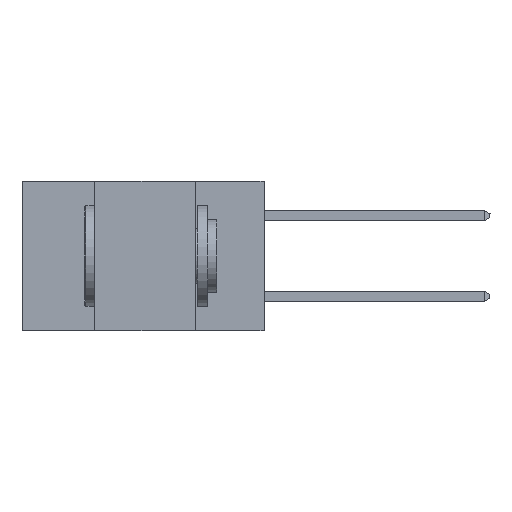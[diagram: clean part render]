
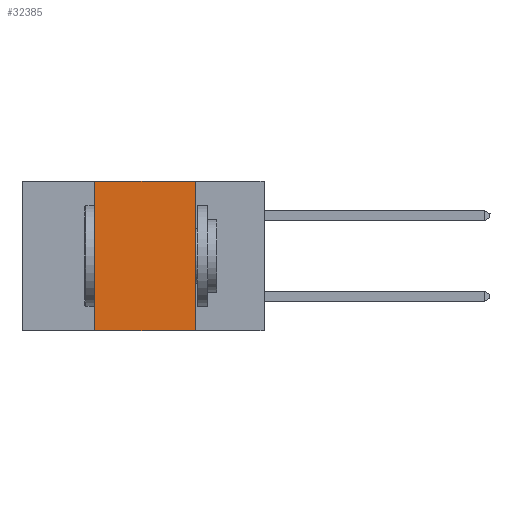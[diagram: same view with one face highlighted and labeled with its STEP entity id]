
A CAD part, left-side view. The second image highlights one B-rep face of the part: STEP entity #32385.
In plain terms, the highlighted planar face has unit normal (-1, 0, 0).
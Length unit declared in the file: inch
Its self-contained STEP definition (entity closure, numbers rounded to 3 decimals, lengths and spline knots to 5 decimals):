
#1073 = AXIS2_PLACEMENT_3D ( 'NONE', #11954, #14558, #14456 ) ;
#1496 = VECTOR ( 'NONE', #25449, 39.37008 ) ;
#1583 = VERTEX_POINT ( 'NONE', #9910 ) ;
#1674 = ORIENTED_EDGE ( 'NONE', *, *, #17111, .F. ) ;
#2244 = DIRECTION ( 'NONE',  ( 0., -1., 0. ) ) ;
#2824 = EDGE_CURVE ( 'NONE', #32663, #30013, #30114, .T. ) ;
#5712 = DIRECTION ( 'NONE',  ( 0., 0., 1. ) ) ;
#8469 = VECTOR ( 'NONE', #2244, 39.37008 ) ;
#8724 = VECTOR ( 'NONE', #5712, 39.37008 ) ;
#9249 = PLANE ( 'NONE',  #1073 ) ;
#9910 = CARTESIAN_POINT ( 'NONE',  ( 0., 0.17, -0.37 ) ) ;
#9993 = ORIENTED_EDGE ( 'NONE', *, *, #13170, .F. ) ;
#10010 = CARTESIAN_POINT ( 'NONE',  ( 0., 0.6, -0.37 ) ) ;
#10573 = CARTESIAN_POINT ( 'NONE',  ( 0., 0.6, 0. ) ) ;
#11084 = ORIENTED_EDGE ( 'NONE', *, *, #2824, .F. ) ;
#11954 = CARTESIAN_POINT ( 'NONE',  ( 0., 0.6, 0. ) ) ;
#13170 = EDGE_CURVE ( 'NONE', #18809, #1583, #32560, .T. ) ;
#14099 = CARTESIAN_POINT ( 'NONE',  ( 0., 0.42, 0. ) ) ;
#14456 = DIRECTION ( 'NONE',  ( 0., 0., -1. ) ) ;
#14558 = DIRECTION ( 'NONE',  ( 1., 0., 0. ) ) ;
#15313 = CARTESIAN_POINT ( 'NONE',  ( 0., 0.42, -0.37 ) ) ;
#15388 = CARTESIAN_POINT ( 'NONE',  ( 0., 0.17, 0. ) ) ;
#17111 = EDGE_CURVE ( 'NONE', #30013, #18809, #28740, .T. ) ;
#17752 = LINE ( 'NONE', #10010, #8469 ) ;
#18809 = VERTEX_POINT ( 'NONE', #15388 ) ;
#20160 = CARTESIAN_POINT ( 'NONE',  ( 0., 0.17, 0. ) ) ;
#21142 = CARTESIAN_POINT ( 'NONE',  ( 0., 0.42, 0. ) ) ;
#23070 = VECTOR ( 'NONE', #31188, 39.37008 ) ;
#25449 = DIRECTION ( 'NONE',  ( 0., 0., -1. ) ) ;
#25602 = FACE_OUTER_BOUND ( 'NONE', #32151, .T. ) ;
#28740 = LINE ( 'NONE', #10573, #23070 ) ;
#29570 = EDGE_CURVE ( 'NONE', #32663, #1583, #17752, .T. ) ;
#30013 = VERTEX_POINT ( 'NONE', #14099 ) ;
#30114 = LINE ( 'NONE', #21142, #8724 ) ;
#31188 = DIRECTION ( 'NONE',  ( 0., -1., 0. ) ) ;
#31572 = ORIENTED_EDGE ( 'NONE', *, *, #29570, .T. ) ;
#32151 = EDGE_LOOP ( 'NONE', ( #9993, #1674, #11084, #31572 ) ) ;
#32385 = ADVANCED_FACE ( 'NONE', ( #25602 ), #9249, .F. ) ;
#32560 = LINE ( 'NONE', #20160, #1496 ) ;
#32663 = VERTEX_POINT ( 'NONE', #15313 ) ;
